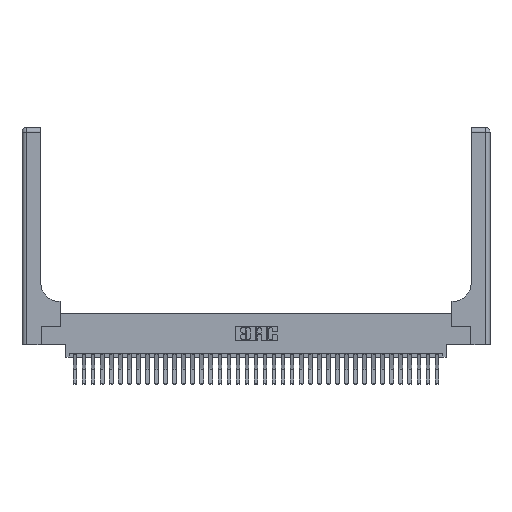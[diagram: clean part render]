
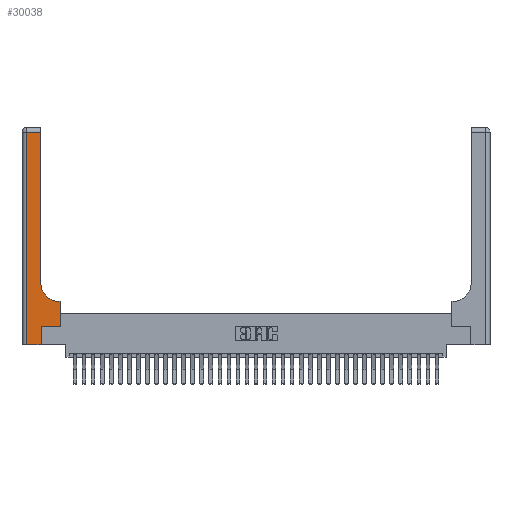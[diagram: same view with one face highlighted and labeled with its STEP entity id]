
A CAD part, top view. The second image highlights one B-rep face of the part: STEP entity #30038.
In plain terms, the highlighted planar face has unit normal (0, 0, 1).
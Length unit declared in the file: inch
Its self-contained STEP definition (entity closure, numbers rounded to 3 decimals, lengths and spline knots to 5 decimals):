
#687 = DIRECTION ( 'NONE',  ( 1., 0., 0. ) ) ;
#1822 = VERTEX_POINT ( 'NONE', #2201 ) ;
#2037 = EDGE_CURVE ( 'NONE', #4431, #19539, #30254, .T. ) ;
#2201 = CARTESIAN_POINT ( 'NONE',  ( 0.265, 0., 0.37 ) ) ;
#3146 = CARTESIAN_POINT ( 'NONE',  ( 0., 3., 0.37 ) ) ;
#4431 = VERTEX_POINT ( 'NONE', #22880 ) ;
#4482 = VECTOR ( 'NONE', #12929, 39.37008 ) ;
#5006 = VERTEX_POINT ( 'NONE', #13062 ) ;
#5317 = EDGE_CURVE ( 'NONE', #1822, #5006, #17478, .T. ) ;
#5662 = DIRECTION ( 'NONE',  ( -1., 0., 0. ) ) ;
#5775 = CARTESIAN_POINT ( 'NONE',  ( 0., 2.94, 0.37 ) ) ;
#6442 = EDGE_CURVE ( 'NONE', #19539, #25316, #14728, .T. ) ;
#6678 = CARTESIAN_POINT ( 'NONE',  ( 0.265, 0., 0.37 ) ) ;
#6876 = ORIENTED_EDGE ( 'NONE', *, *, #19205, .T. ) ;
#7147 = EDGE_CURVE ( 'NONE', #28607, #26416, #9310, .T. ) ;
#7249 = ORIENTED_EDGE ( 'NONE', *, *, #15851, .T. ) ;
#7278 = FACE_OUTER_BOUND ( 'NONE', #17005, .T. ) ;
#8167 = CARTESIAN_POINT ( 'NONE',  ( 0.06, 2.94, 0.37 ) ) ;
#8169 = VECTOR ( 'NONE', #13350, 39.37008 ) ;
#8310 = EDGE_CURVE ( 'NONE', #26416, #9656, #15275, .T. ) ;
#8493 = CARTESIAN_POINT ( 'NONE',  ( 0.51, 0.6, 0.37 ) ) ;
#9137 = CARTESIAN_POINT ( 'NONE',  ( 0.528, 0.25, 0.37 ) ) ;
#9310 = LINE ( 'NONE', #9137, #20898 ) ;
#9656 = VERTEX_POINT ( 'NONE', #8493 ) ;
#10545 = PLANE ( 'NONE',  #24408 ) ;
#11097 = CARTESIAN_POINT ( 'NONE',  ( 0.26, 0.6, 0.37 ) ) ;
#11499 = ORIENTED_EDGE ( 'NONE', *, *, #2037, .T. ) ;
#11675 = CARTESIAN_POINT ( 'NONE',  ( 0.06, 0., 0.37 ) ) ;
#11690 = VECTOR ( 'NONE', #24055, 39.37008 ) ;
#12929 = DIRECTION ( 'NONE',  ( 0., 1., 0. ) ) ;
#13062 = CARTESIAN_POINT ( 'NONE',  ( 0.265, 0.25, 0.37 ) ) ;
#13350 = DIRECTION ( 'NONE',  ( -1., 0., 0. ) ) ;
#14123 = CARTESIAN_POINT ( 'NONE',  ( 0.26, 2.94, 0.37 ) ) ;
#14728 = LINE ( 'NONE', #5775, #8169 ) ;
#15275 = LINE ( 'NONE', #11097, #17584 ) ;
#15352 = ORIENTED_EDGE ( 'NONE', *, *, #19250, .T. ) ;
#15537 = LINE ( 'NONE', #22104, #21381 ) ;
#15541 = DIRECTION ( 'NONE',  ( 0., 0., -1. ) ) ;
#15650 = CARTESIAN_POINT ( 'NONE',  ( 0., 0., 0.37 ) ) ;
#15851 = EDGE_CURVE ( 'NONE', #25316, #19516, #18807, .T. ) ;
#15923 = LINE ( 'NONE', #15650, #28459 ) ;
#16065 = DIRECTION ( 'NONE',  ( -1., 0., 0. ) ) ;
#16938 = ORIENTED_EDGE ( 'NONE', *, *, #7147, .T. ) ;
#17005 = EDGE_LOOP ( 'NONE', ( #11499, #19633, #7249, #15352, #28669, #29478, #16938, #23548, #6876 ) ) ;
#17478 = LINE ( 'NONE', #6678, #11690 ) ;
#17584 = VECTOR ( 'NONE', #16065, 39.37008 ) ;
#18160 = DIRECTION ( 'NONE',  ( 1., 0., 0. ) ) ;
#18807 = LINE ( 'NONE', #31921, #25493 ) ;
#19053 = EDGE_CURVE ( 'NONE', #5006, #28607, #15537, .T. ) ;
#19205 = EDGE_CURVE ( 'NONE', #9656, #4431, #30847, .T. ) ;
#19250 = EDGE_CURVE ( 'NONE', #19516, #1822, #15923, .T. ) ;
#19516 = VERTEX_POINT ( 'NONE', #11675 ) ;
#19539 = VERTEX_POINT ( 'NONE', #14123 ) ;
#19633 = ORIENTED_EDGE ( 'NONE', *, *, #6442, .T. ) ;
#19813 = CARTESIAN_POINT ( 'NONE',  ( 0.528, 0.25, 0.37 ) ) ;
#20389 = CARTESIAN_POINT ( 'NONE',  ( 0.26, 3., 0.37 ) ) ;
#20506 = DIRECTION ( 'NONE',  ( 0., 0., -1. ) ) ;
#20898 = VECTOR ( 'NONE', #28944, 39.37008 ) ;
#21381 = VECTOR ( 'NONE', #24651, 39.37008 ) ;
#22104 = CARTESIAN_POINT ( 'NONE',  ( 0.265, 0.25, 0.37 ) ) ;
#22880 = CARTESIAN_POINT ( 'NONE',  ( 0.26, 0.85, 0.37 ) ) ;
#23548 = ORIENTED_EDGE ( 'NONE', *, *, #8310, .T. ) ;
#24055 = DIRECTION ( 'NONE',  ( 0., 1., 0. ) ) ;
#24303 = DIRECTION ( 'NONE',  ( 0., -1., 0. ) ) ;
#24408 = AXIS2_PLACEMENT_3D ( 'NONE', #3146, #20506, #5662 ) ;
#24651 = DIRECTION ( 'NONE',  ( 1., 0., 0. ) ) ;
#25316 = VERTEX_POINT ( 'NONE', #8167 ) ;
#25493 = VECTOR ( 'NONE', #24303, 39.37008 ) ;
#26416 = VERTEX_POINT ( 'NONE', #31063 ) ;
#26535 = AXIS2_PLACEMENT_3D ( 'NONE', #30579, #15541, #687 ) ;
#28459 = VECTOR ( 'NONE', #18160, 39.37008 ) ;
#28607 = VERTEX_POINT ( 'NONE', #19813 ) ;
#28669 = ORIENTED_EDGE ( 'NONE', *, *, #5317, .T. ) ;
#28944 = DIRECTION ( 'NONE',  ( 0., 1., 0. ) ) ;
#29478 = ORIENTED_EDGE ( 'NONE', *, *, #19053, .T. ) ;
#30038 = ADVANCED_FACE ( 'NONE', ( #7278 ), #10545, .F. ) ;
#30254 = LINE ( 'NONE', #20389, #4482 ) ;
#30579 = CARTESIAN_POINT ( 'NONE',  ( 0.51, 0.85, 0.37 ) ) ;
#30847 = CIRCLE ( 'NONE', #26535, 0.25 ) ;
#31063 = CARTESIAN_POINT ( 'NONE',  ( 0.528, 0.6, 0.37 ) ) ;
#31921 = CARTESIAN_POINT ( 'NONE',  ( 0.06, 3., 0.37 ) ) ;
